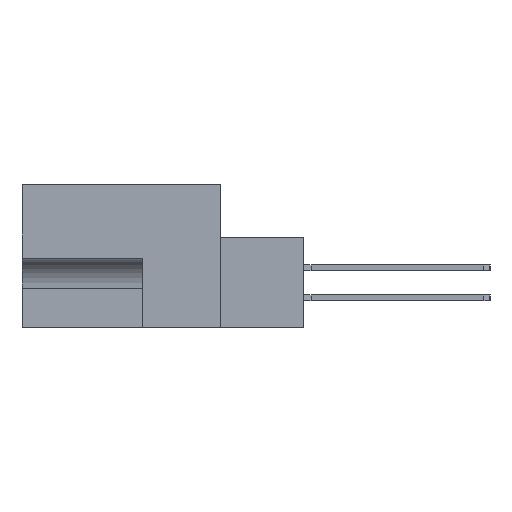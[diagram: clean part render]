
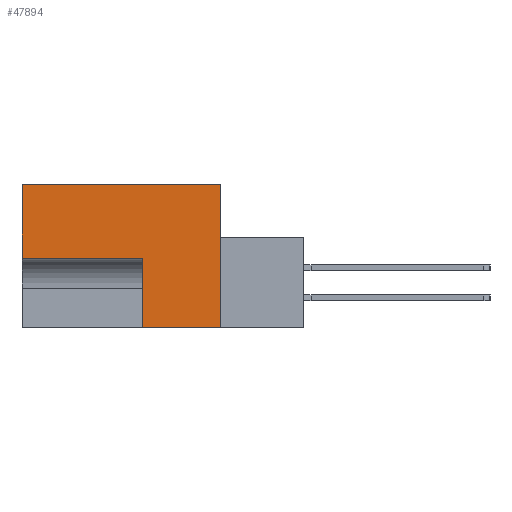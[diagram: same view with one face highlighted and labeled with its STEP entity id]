
A CAD part, left-side view. The second image highlights one B-rep face of the part: STEP entity #47894.
In plain terms, the highlighted planar face has unit normal (-1, 0, 0).
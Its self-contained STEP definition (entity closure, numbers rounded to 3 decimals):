
#847 = EDGE_CURVE ( 'NONE', #33022, #28525, #20053, .T. ) ;
#2055 = ORIENTED_EDGE ( 'NONE', *, *, #10370, .F. ) ;
#3113 = CARTESIAN_POINT ( 'NONE',  ( 0., 8.255, -15.088 ) ) ;
#3767 = DIRECTION ( 'NONE',  ( 0., -1., 0. ) ) ;
#4887 = CARTESIAN_POINT ( 'NONE',  ( 0., 0., 0. ) ) ;
#5492 = EDGE_CURVE ( 'NONE', #37353, #20212, #37016, .T. ) ;
#8131 = CARTESIAN_POINT ( 'NONE',  ( 0., 11.506, 0. ) ) ;
#8658 = ORIENTED_EDGE ( 'NONE', *, *, #25695, .F. ) ;
#9083 = LINE ( 'NONE', #49297, #27831 ) ;
#9189 = CARTESIAN_POINT ( 'NONE',  ( 0., 0., -15.088 ) ) ;
#9825 = FACE_OUTER_BOUND ( 'NONE', #28859, .T. ) ;
#10160 = LINE ( 'NONE', #43244, #51397 ) ;
#10370 = EDGE_CURVE ( 'NONE', #22900, #37353, #47900, .T. ) ;
#10455 = EDGE_CURVE ( 'NONE', #20212, #33022, #9083, .T. ) ;
#12192 = ORIENTED_EDGE ( 'NONE', *, *, #5492, .F. ) ;
#14618 = DIRECTION ( 'NONE',  ( 0., 0., -1. ) ) ;
#15156 = DIRECTION ( 'NONE',  ( 0., 0., 1. ) ) ;
#15799 = CARTESIAN_POINT ( 'NONE',  ( 0., 20.955, -15.088 ) ) ;
#16055 = CARTESIAN_POINT ( 'NONE',  ( 0., 20.955, 0. ) ) ;
#16886 = CARTESIAN_POINT ( 'NONE',  ( 0., 8.255, -7.772 ) ) ;
#19755 = DIRECTION ( 'NONE',  ( 0., 0., 1. ) ) ;
#20053 = LINE ( 'NONE', #49397, #43198 ) ;
#20212 = VERTEX_POINT ( 'NONE', #4887 ) ;
#21552 = DIRECTION ( 'NONE',  ( 0., 1., 0. ) ) ;
#22900 = VERTEX_POINT ( 'NONE', #28071 ) ;
#24112 = AXIS2_PLACEMENT_3D ( 'NONE', #38512, #50240, #14618 ) ;
#25695 = EDGE_CURVE ( 'NONE', #49291, #22900, #26700, .T. ) ;
#26700 = LINE ( 'NONE', #42143, #37306 ) ;
#27076 = VECTOR ( 'NONE', #3767, 1000. ) ;
#27831 = VECTOR ( 'NONE', #32676, 1000. ) ;
#28071 = CARTESIAN_POINT ( 'NONE',  ( 0., 20.955, -7.772 ) ) ;
#28525 = VERTEX_POINT ( 'NONE', #3113 ) ;
#28859 = EDGE_LOOP ( 'NONE', ( #33330, #38713, #12192, #2055, #8658, #37739 ) ) ;
#29132 = EDGE_CURVE ( 'NONE', #28525, #49291, #10160, .T. ) ;
#32676 = DIRECTION ( 'NONE',  ( 0., 0., -1. ) ) ;
#33022 = VERTEX_POINT ( 'NONE', #9189 ) ;
#33330 = ORIENTED_EDGE ( 'NONE', *, *, #847, .F. ) ;
#37016 = LINE ( 'NONE', #8131, #27076 ) ;
#37254 = VECTOR ( 'NONE', #19755, 1000. ) ;
#37306 = VECTOR ( 'NONE', #21552, 1000. ) ;
#37353 = VERTEX_POINT ( 'NONE', #16055 ) ;
#37739 = ORIENTED_EDGE ( 'NONE', *, *, #29132, .F. ) ;
#38512 = CARTESIAN_POINT ( 'NONE',  ( 0., 0., 0. ) ) ;
#38713 = ORIENTED_EDGE ( 'NONE', *, *, #10455, .F. ) ;
#40978 = DIRECTION ( 'NONE',  ( 0., 1., 0. ) ) ;
#42143 = CARTESIAN_POINT ( 'NONE',  ( 0., 8.255, -7.772 ) ) ;
#43198 = VECTOR ( 'NONE', #40978, 1000. ) ;
#43244 = CARTESIAN_POINT ( 'NONE',  ( 0., 8.255, -15.088 ) ) ;
#46242 = PLANE ( 'NONE',  #24112 ) ;
#47894 = ADVANCED_FACE ( 'NONE', ( #9825 ), #46242, .F. ) ;
#47900 = LINE ( 'NONE', #15799, #37254 ) ;
#49291 = VERTEX_POINT ( 'NONE', #16886 ) ;
#49297 = CARTESIAN_POINT ( 'NONE',  ( 0., 0., 0. ) ) ;
#49397 = CARTESIAN_POINT ( 'NONE',  ( 0., -8.814, -15.088 ) ) ;
#50240 = DIRECTION ( 'NONE',  ( 1., 0., 0. ) ) ;
#51397 = VECTOR ( 'NONE', #15156, 1000. ) ;
